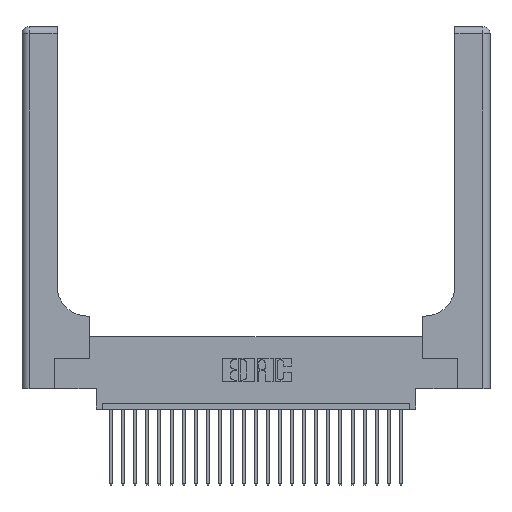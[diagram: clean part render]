
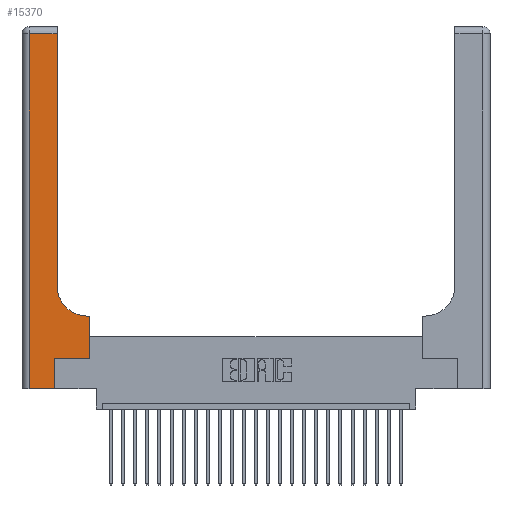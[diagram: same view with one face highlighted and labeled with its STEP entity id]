
A CAD part, top view. The second image highlights one B-rep face of the part: STEP entity #15370.
In plain terms, the highlighted planar face has unit normal (0, 0, 1).
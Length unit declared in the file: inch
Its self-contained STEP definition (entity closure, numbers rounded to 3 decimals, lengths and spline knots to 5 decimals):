
#14 = CARTESIAN_POINT ( 'NONE',  ( 0.269, 0., 0.37 ) ) ;
#524 = LINE ( 'NONE', #9961, #13633 ) ;
#610 = ORIENTED_EDGE ( 'NONE', *, *, #25148, .T. ) ;
#761 = VECTOR ( 'NONE', #24732, 39.37008 ) ;
#830 = ORIENTED_EDGE ( 'NONE', *, *, #25821, .T. ) ;
#952 = DIRECTION ( 'NONE',  ( 1., 0., 0. ) ) ;
#1487 = DIRECTION ( 'NONE',  ( 0., 1., 0. ) ) ;
#1893 = VERTEX_POINT ( 'NONE', #16786 ) ;
#2119 = CARTESIAN_POINT ( 'NONE',  ( 0.2915, 0.6, 0.37 ) ) ;
#3531 = EDGE_CURVE ( 'NONE', #14508, #13237, #12887, .T. ) ;
#3661 = VECTOR ( 'NONE', #20128, 39.37008 ) ;
#4287 = LINE ( 'NONE', #24470, #3661 ) ;
#4831 = VECTOR ( 'NONE', #7366, 39.37008 ) ;
#4978 = DIRECTION ( 'NONE',  ( -1., 0., 0. ) ) ;
#5081 = CARTESIAN_POINT ( 'NONE',  ( 0.5585, 0.25, 0.37 ) ) ;
#5313 = EDGE_CURVE ( 'NONE', #15182, #14508, #15107, .T. ) ;
#5454 = DIRECTION ( 'NONE',  ( 0., -1., 0. ) ) ;
#5657 = FACE_OUTER_BOUND ( 'NONE', #9779, .T. ) ;
#5708 = DIRECTION ( 'NONE',  ( 0., 1., 0. ) ) ;
#6561 = LINE ( 'NONE', #23789, #8463 ) ;
#7366 = DIRECTION ( 'NONE',  ( 0., 1., 0. ) ) ;
#7840 = VERTEX_POINT ( 'NONE', #16240 ) ;
#8463 = VECTOR ( 'NONE', #5454, 39.37008 ) ;
#9043 = CARTESIAN_POINT ( 'NONE',  ( 0.5415, 0.6, 0.37 ) ) ;
#9734 = CARTESIAN_POINT ( 'NONE',  ( 0.5585, 0.6, 0.37 ) ) ;
#9779 = EDGE_LOOP ( 'NONE', ( #21907, #24522, #26020, #11804, #17896, #830, #15772, #610, #13624 ) ) ;
#9961 = CARTESIAN_POINT ( 'NONE',  ( 0.5585, 0.25, 0.37 ) ) ;
#10194 = LINE ( 'NONE', #14, #4831 ) ;
#10595 = EDGE_CURVE ( 'NONE', #13237, #16560, #6561, .T. ) ;
#10778 = CARTESIAN_POINT ( 'NONE',  ( 0., 2.94, 0.37 ) ) ;
#10992 = CARTESIAN_POINT ( 'NONE',  ( 0.2915, 0.85, 0.37 ) ) ;
#11131 = EDGE_CURVE ( 'NONE', #16560, #1893, #4287, .T. ) ;
#11731 = LINE ( 'NONE', #2119, #20652 ) ;
#11804 = ORIENTED_EDGE ( 'NONE', *, *, #11131, .T. ) ;
#12211 = EDGE_CURVE ( 'NONE', #18899, #15182, #19218, .T. ) ;
#12887 = LINE ( 'NONE', #10778, #761 ) ;
#13237 = VERTEX_POINT ( 'NONE', #17254 ) ;
#13624 = ORIENTED_EDGE ( 'NONE', *, *, #12211, .T. ) ;
#13633 = VECTOR ( 'NONE', #5708, 39.37008 ) ;
#14228 = CARTESIAN_POINT ( 'NONE',  ( 0.269, 0.25, 0.37 ) ) ;
#14508 = VERTEX_POINT ( 'NONE', #15557 ) ;
#15107 = LINE ( 'NONE', #17762, #20491 ) ;
#15182 = VERTEX_POINT ( 'NONE', #10992 ) ;
#15370 = ADVANCED_FACE ( 'NONE', ( #5657 ), #22963, .F. ) ;
#15557 = CARTESIAN_POINT ( 'NONE',  ( 0.2915, 2.94, 0.37 ) ) ;
#15772 = ORIENTED_EDGE ( 'NONE', *, *, #25619, .T. ) ;
#16240 = CARTESIAN_POINT ( 'NONE',  ( 0.269, 0.25, 0.37 ) ) ;
#16560 = VERTEX_POINT ( 'NONE', #20106 ) ;
#16786 = CARTESIAN_POINT ( 'NONE',  ( 0.269, 0., 0.37 ) ) ;
#17227 = CARTESIAN_POINT ( 'NONE',  ( 0.5415, 0.85, 0.37 ) ) ;
#17254 = CARTESIAN_POINT ( 'NONE',  ( 0.06, 2.94, 0.37 ) ) ;
#17762 = CARTESIAN_POINT ( 'NONE',  ( 0.2915, 3., 0.37 ) ) ;
#17896 = ORIENTED_EDGE ( 'NONE', *, *, #18169, .T. ) ;
#18169 = EDGE_CURVE ( 'NONE', #1893, #7840, #10194, .T. ) ;
#18506 = DIRECTION ( 'NONE',  ( 1., 0., 0. ) ) ;
#18899 = VERTEX_POINT ( 'NONE', #9043 ) ;
#18998 = VERTEX_POINT ( 'NONE', #9734 ) ;
#19218 = CIRCLE ( 'NONE', #19256, 0.25 ) ;
#19256 = AXIS2_PLACEMENT_3D ( 'NONE', #17227, #25480, #952 ) ;
#20106 = CARTESIAN_POINT ( 'NONE',  ( 0.06, 0., 0.37 ) ) ;
#20128 = DIRECTION ( 'NONE',  ( 1., 0., 0. ) ) ;
#20240 = AXIS2_PLACEMENT_3D ( 'NONE', #25000, #21028, #4978 ) ;
#20411 = DIRECTION ( 'NONE',  ( -1., 0., 0. ) ) ;
#20491 = VECTOR ( 'NONE', #1487, 39.37008 ) ;
#20652 = VECTOR ( 'NONE', #20411, 39.37008 ) ;
#21028 = DIRECTION ( 'NONE',  ( 0., 0., -1. ) ) ;
#21907 = ORIENTED_EDGE ( 'NONE', *, *, #5313, .T. ) ;
#22558 = LINE ( 'NONE', #14228, #26407 ) ;
#22963 = PLANE ( 'NONE',  #20240 ) ;
#23730 = VERTEX_POINT ( 'NONE', #5081 ) ;
#23789 = CARTESIAN_POINT ( 'NONE',  ( 0.06, 3., 0.37 ) ) ;
#24470 = CARTESIAN_POINT ( 'NONE',  ( 0., 0., 0.37 ) ) ;
#24522 = ORIENTED_EDGE ( 'NONE', *, *, #3531, .T. ) ;
#24732 = DIRECTION ( 'NONE',  ( -1., 0., 0. ) ) ;
#25000 = CARTESIAN_POINT ( 'NONE',  ( 0., 3., 0.37 ) ) ;
#25148 = EDGE_CURVE ( 'NONE', #18998, #18899, #11731, .T. ) ;
#25480 = DIRECTION ( 'NONE',  ( 0., 0., -1. ) ) ;
#25619 = EDGE_CURVE ( 'NONE', #23730, #18998, #524, .T. ) ;
#25821 = EDGE_CURVE ( 'NONE', #7840, #23730, #22558, .T. ) ;
#26020 = ORIENTED_EDGE ( 'NONE', *, *, #10595, .T. ) ;
#26407 = VECTOR ( 'NONE', #18506, 39.37008 ) ;
